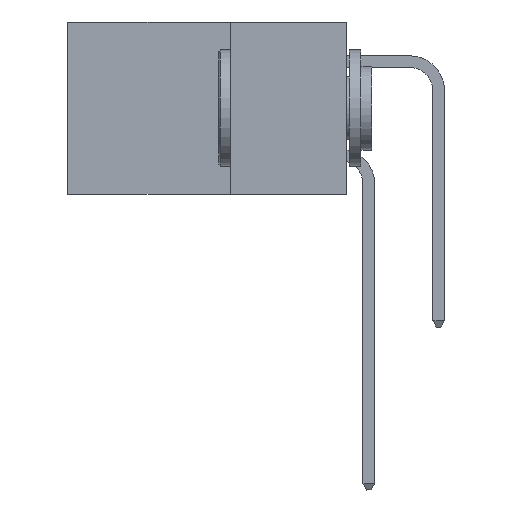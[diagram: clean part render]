
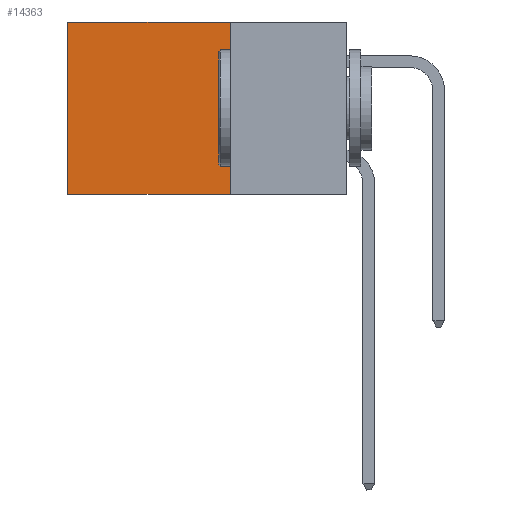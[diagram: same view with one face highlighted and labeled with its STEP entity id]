
A CAD part, left-side view. The second image highlights one B-rep face of the part: STEP entity #14363.
In plain terms, the highlighted planar face has unit normal (-1, 0, 0).
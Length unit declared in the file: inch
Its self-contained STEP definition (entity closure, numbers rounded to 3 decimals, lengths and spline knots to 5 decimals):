
#121 = VECTOR ( 'NONE', #10126, 39.37008 ) ;
#746 = CARTESIAN_POINT ( 'NONE',  ( 0.2875, 0.25, -0.37 ) ) ;
#1442 = CARTESIAN_POINT ( 'NONE',  ( 0.2875, 0.25, 0. ) ) ;
#2588 = VECTOR ( 'NONE', #9831, 39.37008 ) ;
#3684 = EDGE_LOOP ( 'NONE', ( #24997, #18534, #16005, #20880 ) ) ;
#3720 = EDGE_CURVE ( 'NONE', #25507, #22199, #15396, .T. ) ;
#3721 = CARTESIAN_POINT ( 'NONE',  ( 0.2875, 0.25, 0. ) ) ;
#4437 = LINE ( 'NONE', #16879, #23054 ) ;
#8423 = DIRECTION ( 'NONE',  ( 0., 1., 0. ) ) ;
#8638 = CARTESIAN_POINT ( 'NONE',  ( 0.2875, 0.25, 0. ) ) ;
#8953 = FACE_OUTER_BOUND ( 'NONE', #3684, .T. ) ;
#9610 = CARTESIAN_POINT ( 'NONE',  ( 0.2875, 0.6, 0. ) ) ;
#9831 = DIRECTION ( 'NONE',  ( 0., 1., 0. ) ) ;
#10126 = DIRECTION ( 'NONE',  ( 0., 0., -1. ) ) ;
#11416 = LINE ( 'NONE', #1442, #121 ) ;
#11443 = VERTEX_POINT ( 'NONE', #9610 ) ;
#11633 = DIRECTION ( 'NONE',  ( 1., 0., 0. ) ) ;
#12197 = EDGE_CURVE ( 'NONE', #11443, #22199, #4437, .T. ) ;
#12482 = CARTESIAN_POINT ( 'NONE',  ( 0.2875, 0.6, -0.37 ) ) ;
#14083 = CARTESIAN_POINT ( 'NONE',  ( 0.2875, 0.25, -0.37 ) ) ;
#14363 = ADVANCED_FACE ( 'NONE', ( #8953 ), #22113, .F. ) ;
#14473 = DIRECTION ( 'NONE',  ( 0., 0., -1. ) ) ;
#14518 = DIRECTION ( 'NONE',  ( 0., 0., -1. ) ) ;
#15396 = LINE ( 'NONE', #14083, #19382 ) ;
#16005 = ORIENTED_EDGE ( 'NONE', *, *, #17749, .F. ) ;
#16738 = CARTESIAN_POINT ( 'NONE',  ( 0.2875, 0.25, 0. ) ) ;
#16879 = CARTESIAN_POINT ( 'NONE',  ( 0.2875, 0.6, 0. ) ) ;
#17749 = EDGE_CURVE ( 'NONE', #25197, #25507, #11416, .T. ) ;
#18534 = ORIENTED_EDGE ( 'NONE', *, *, #3720, .F. ) ;
#19382 = VECTOR ( 'NONE', #8423, 39.37008 ) ;
#20880 = ORIENTED_EDGE ( 'NONE', *, *, #23382, .T. ) ;
#22113 = PLANE ( 'NONE',  #27244 ) ;
#22199 = VERTEX_POINT ( 'NONE', #12482 ) ;
#23054 = VECTOR ( 'NONE', #14518, 39.37008 ) ;
#23382 = EDGE_CURVE ( 'NONE', #25197, #11443, #26144, .T. ) ;
#24997 = ORIENTED_EDGE ( 'NONE', *, *, #12197, .T. ) ;
#25197 = VERTEX_POINT ( 'NONE', #16738 ) ;
#25507 = VERTEX_POINT ( 'NONE', #746 ) ;
#26144 = LINE ( 'NONE', #3721, #2588 ) ;
#27244 = AXIS2_PLACEMENT_3D ( 'NONE', #8638, #11633, #14473 ) ;
